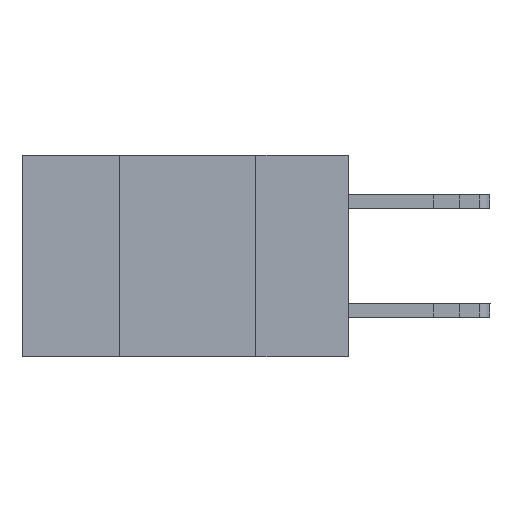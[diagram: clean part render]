
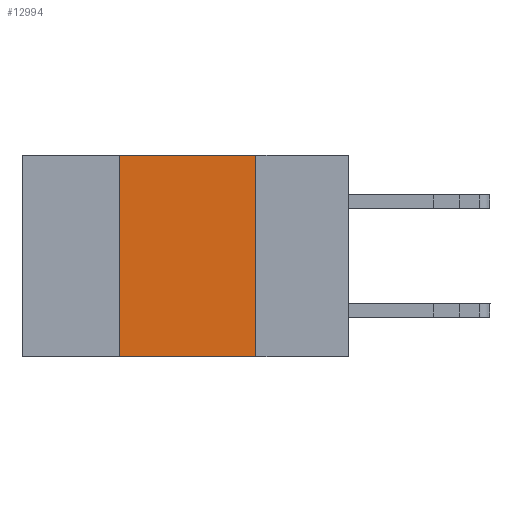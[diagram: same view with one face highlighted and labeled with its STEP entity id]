
A CAD part, left-side view. The second image highlights one B-rep face of the part: STEP entity #12994.
In plain terms, the highlighted planar face has unit normal (-1, 0, 0).
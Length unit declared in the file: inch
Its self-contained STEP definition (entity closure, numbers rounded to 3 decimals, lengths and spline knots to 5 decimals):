
#1407 = EDGE_LOOP ( 'NONE', ( #12416, #12431, #12538, #12563 ) ) ;
#1702 = CARTESIAN_POINT ( 'NONE',  ( 0., 0.17, -0.37 ) ) ;
#2545 = VECTOR ( 'NONE', #5060, 39.37008 ) ;
#2815 = CARTESIAN_POINT ( 'NONE',  ( 0., 0.42, -0.37 ) ) ;
#3028 = VECTOR ( 'NONE', #13780, 39.37008 ) ;
#3768 = CARTESIAN_POINT ( 'NONE',  ( 0., 0.42, 0. ) ) ;
#4122 = CARTESIAN_POINT ( 'NONE',  ( 0., 0.6, 0. ) ) ;
#4611 = VERTEX_POINT ( 'NONE', #14391 ) ;
#4702 = EDGE_CURVE ( 'NONE', #8460, #9182, #11075, .T. ) ;
#4733 = FACE_OUTER_BOUND ( 'NONE', #1407, .T. ) ;
#4887 = EDGE_CURVE ( 'NONE', #9182, #6474, #9041, .T. ) ;
#5060 = DIRECTION ( 'NONE',  ( 0., 0., 1. ) ) ;
#5253 = DIRECTION ( 'NONE',  ( 0., 0., -1. ) ) ;
#5655 = LINE ( 'NONE', #7254, #3028 ) ;
#6474 = VERTEX_POINT ( 'NONE', #1702 ) ;
#7254 = CARTESIAN_POINT ( 'NONE',  ( 0., 0.6, -0.37 ) ) ;
#8460 = VERTEX_POINT ( 'NONE', #3768 ) ;
#8542 = PLANE ( 'NONE',  #12514 ) ;
#9041 = LINE ( 'NONE', #11832, #11246 ) ;
#9182 = VERTEX_POINT ( 'NONE', #11609 ) ;
#10446 = EDGE_CURVE ( 'NONE', #4611, #8460, #11391, .T. ) ;
#11075 = LINE ( 'NONE', #13321, #11422 ) ;
#11246 = VECTOR ( 'NONE', #11895, 39.37008 ) ;
#11391 = LINE ( 'NONE', #2815, #2545 ) ;
#11422 = VECTOR ( 'NONE', #13280, 39.37008 ) ;
#11533 = EDGE_CURVE ( 'NONE', #4611, #6474, #5655, .T. ) ;
#11609 = CARTESIAN_POINT ( 'NONE',  ( 0., 0.17, 0. ) ) ;
#11832 = CARTESIAN_POINT ( 'NONE',  ( 0., 0.17, -0.37 ) ) ;
#11868 = DIRECTION ( 'NONE',  ( 1., 0., 0. ) ) ;
#11895 = DIRECTION ( 'NONE',  ( 0., 0., -1. ) ) ;
#12416 = ORIENTED_EDGE ( 'NONE', *, *, #4887, .F. ) ;
#12431 = ORIENTED_EDGE ( 'NONE', *, *, #4702, .F. ) ;
#12514 = AXIS2_PLACEMENT_3D ( 'NONE', #4122, #11868, #5253 ) ;
#12538 = ORIENTED_EDGE ( 'NONE', *, *, #10446, .F. ) ;
#12563 = ORIENTED_EDGE ( 'NONE', *, *, #11533, .T. ) ;
#12994 = ADVANCED_FACE ( 'NONE', ( #4733 ), #8542, .F. ) ;
#13280 = DIRECTION ( 'NONE',  ( 0., -1., 0. ) ) ;
#13321 = CARTESIAN_POINT ( 'NONE',  ( 0., 0.6, 0. ) ) ;
#13780 = DIRECTION ( 'NONE',  ( 0., -1., 0. ) ) ;
#14391 = CARTESIAN_POINT ( 'NONE',  ( 0., 0.42, -0.37 ) ) ;
